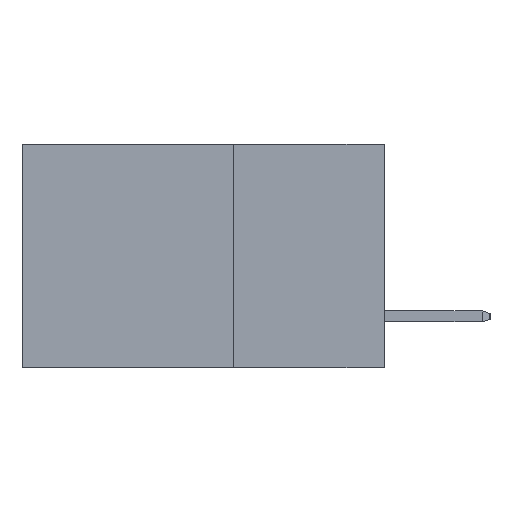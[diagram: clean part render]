
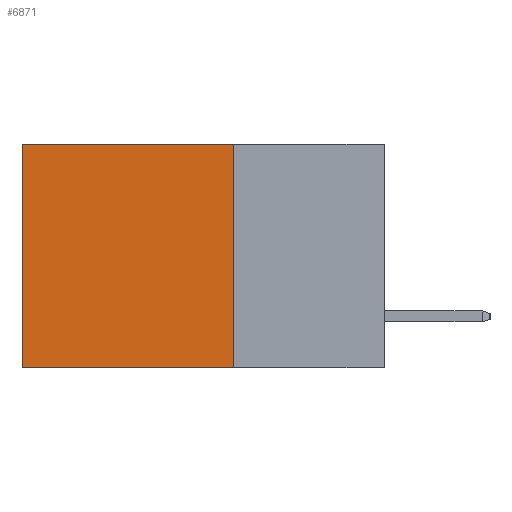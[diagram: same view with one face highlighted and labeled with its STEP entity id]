
A CAD part, left-side view. The second image highlights one B-rep face of the part: STEP entity #6871.
In plain terms, the highlighted planar face has unit normal (-1, 0, 0).
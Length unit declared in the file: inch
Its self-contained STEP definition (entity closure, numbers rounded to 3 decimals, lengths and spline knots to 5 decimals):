
#536 = ORIENTED_EDGE ( 'NONE', *, *, #3642, .F. ) ;
#613 = VERTEX_POINT ( 'NONE', #8699 ) ;
#856 = ORIENTED_EDGE ( 'NONE', *, *, #2393, .T. ) ;
#1275 = VERTEX_POINT ( 'NONE', #8706 ) ;
#2303 = LINE ( 'NONE', #4209, #10067 ) ;
#2352 = DIRECTION ( 'NONE',  ( 1., 0., 0. ) ) ;
#2393 = EDGE_CURVE ( 'NONE', #4308, #8941, #5619, .T. ) ;
#2543 = EDGE_LOOP ( 'NONE', ( #6639, #536, #9515, #856 ) ) ;
#2787 = DIRECTION ( 'NONE',  ( 0., 1., 0. ) ) ;
#3642 = EDGE_CURVE ( 'NONE', #613, #1275, #2303, .T. ) ;
#3797 = DIRECTION ( 'NONE',  ( 0., 0., -1. ) ) ;
#3977 = VECTOR ( 'NONE', #7116, 39.37008 ) ;
#4016 = CARTESIAN_POINT ( 'NONE',  ( 0.298, 0.25, 0. ) ) ;
#4146 = EDGE_CURVE ( 'NONE', #4308, #613, #9306, .T. ) ;
#4209 = CARTESIAN_POINT ( 'NONE',  ( 0.298, 0.25, -0.37 ) ) ;
#4308 = VERTEX_POINT ( 'NONE', #4016 ) ;
#4368 = PLANE ( 'NONE',  #10164 ) ;
#4645 = CARTESIAN_POINT ( 'NONE',  ( 0.298, 0.25, 0. ) ) ;
#5061 = CARTESIAN_POINT ( 'NONE',  ( 0.298, 0.6, 0. ) ) ;
#5619 = LINE ( 'NONE', #7102, #3977 ) ;
#5830 = CARTESIAN_POINT ( 'NONE',  ( 0.298, 0.25, 0. ) ) ;
#6048 = FACE_OUTER_BOUND ( 'NONE', #2543, .T. ) ;
#6201 = DIRECTION ( 'NONE',  ( 0., 0., -1. ) ) ;
#6436 = EDGE_CURVE ( 'NONE', #8941, #1275, #8158, .T. ) ;
#6639 = ORIENTED_EDGE ( 'NONE', *, *, #6436, .T. ) ;
#6871 = ADVANCED_FACE ( 'NONE', ( #6048 ), #4368, .F. ) ;
#7102 = CARTESIAN_POINT ( 'NONE',  ( 0.298, 0.25, 0. ) ) ;
#7116 = DIRECTION ( 'NONE',  ( 0., 1., 0. ) ) ;
#8158 = LINE ( 'NONE', #10285, #10259 ) ;
#8425 = DIRECTION ( 'NONE',  ( 0., 0., -1. ) ) ;
#8699 = CARTESIAN_POINT ( 'NONE',  ( 0.298, 0.25, -0.37 ) ) ;
#8706 = CARTESIAN_POINT ( 'NONE',  ( 0.298, 0.6, -0.37 ) ) ;
#8941 = VERTEX_POINT ( 'NONE', #5061 ) ;
#9076 = VECTOR ( 'NONE', #8425, 39.37008 ) ;
#9306 = LINE ( 'NONE', #4645, #9076 ) ;
#9515 = ORIENTED_EDGE ( 'NONE', *, *, #4146, .F. ) ;
#10067 = VECTOR ( 'NONE', #2787, 39.37008 ) ;
#10164 = AXIS2_PLACEMENT_3D ( 'NONE', #5830, #2352, #6201 ) ;
#10259 = VECTOR ( 'NONE', #3797, 39.37008 ) ;
#10285 = CARTESIAN_POINT ( 'NONE',  ( 0.298, 0.6, 0. ) ) ;
